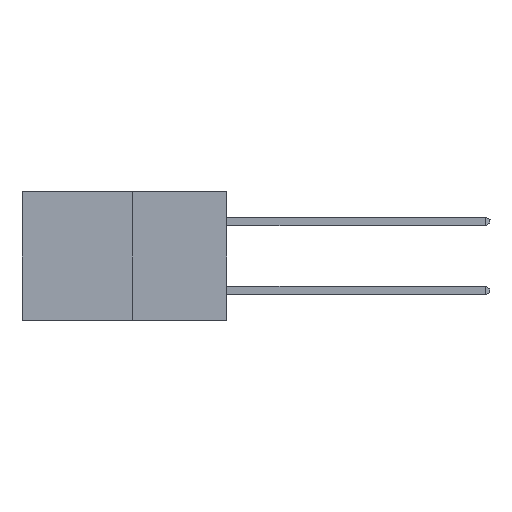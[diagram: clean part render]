
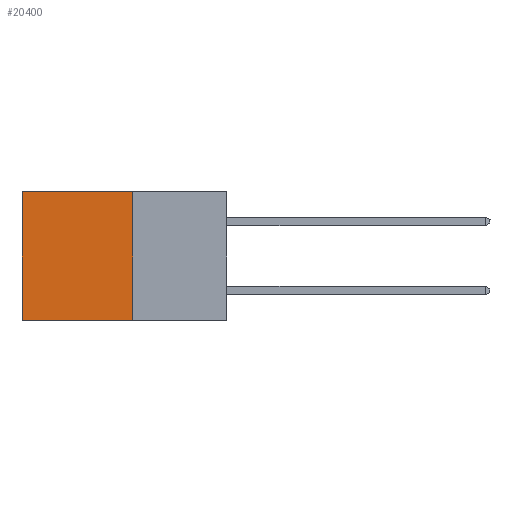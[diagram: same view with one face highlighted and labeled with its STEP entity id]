
A CAD part, left-side view. The second image highlights one B-rep face of the part: STEP entity #20400.
In plain terms, the highlighted planar face has unit normal (-1, 0, 0).
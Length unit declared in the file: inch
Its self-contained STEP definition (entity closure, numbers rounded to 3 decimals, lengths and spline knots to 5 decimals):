
#380 = CARTESIAN_POINT ( 'NONE',  ( 0.277, 0.27, -0.37 ) ) ;
#531 = VERTEX_POINT ( 'NONE', #34738 ) ;
#3915 = EDGE_CURVE ( 'NONE', #531, #27552, #3967, .T. ) ;
#3924 = ORIENTED_EDGE ( 'NONE', *, *, #5688, .T. ) ;
#3967 = LINE ( 'NONE', #10263, #10322 ) ;
#5487 = ORIENTED_EDGE ( 'NONE', *, *, #3915, .F. ) ;
#5511 = CARTESIAN_POINT ( 'NONE',  ( 0.277, 0.27, -0.37 ) ) ;
#5688 = EDGE_CURVE ( 'NONE', #26349, #24792, #20403, .T. ) ;
#5805 = EDGE_CURVE ( 'NONE', #531, #26349, #30429, .T. ) ;
#7483 = VECTOR ( 'NONE', #22074, 39.37008 ) ;
#9170 = LINE ( 'NONE', #380, #7483 ) ;
#9884 = CARTESIAN_POINT ( 'NONE',  ( 0.277, 0.27, 0. ) ) ;
#9928 = DIRECTION ( 'NONE',  ( 0., 1., 0. ) ) ;
#10263 = CARTESIAN_POINT ( 'NONE',  ( 0.277, 0.27, -0.37 ) ) ;
#10322 = VECTOR ( 'NONE', #28359, 39.37008 ) ;
#10988 = ORIENTED_EDGE ( 'NONE', *, *, #33969, .F. ) ;
#15325 = PLANE ( 'NONE',  #32573 ) ;
#16840 = DIRECTION ( 'NONE',  ( 0., 0., -1. ) ) ;
#17009 = VECTOR ( 'NONE', #9928, 39.37008 ) ;
#17057 = CARTESIAN_POINT ( 'NONE',  ( 0.277, 0.59, -0.37 ) ) ;
#18037 = DIRECTION ( 'NONE',  ( 0., 0., -1. ) ) ;
#19739 = CARTESIAN_POINT ( 'NONE',  ( 0.277, 0.59, 0. ) ) ;
#20400 = ADVANCED_FACE ( 'NONE', ( #21377 ), #15325, .F. ) ;
#20403 = LINE ( 'NONE', #17057, #33793 ) ;
#21377 = FACE_OUTER_BOUND ( 'NONE', #26515, .T. ) ;
#22074 = DIRECTION ( 'NONE',  ( 0., 1., 0. ) ) ;
#24358 = ORIENTED_EDGE ( 'NONE', *, *, #5805, .T. ) ;
#24792 = VERTEX_POINT ( 'NONE', #32463 ) ;
#25948 = CARTESIAN_POINT ( 'NONE',  ( 0.277, 0.27, -0.37 ) ) ;
#26349 = VERTEX_POINT ( 'NONE', #19739 ) ;
#26515 = EDGE_LOOP ( 'NONE', ( #3924, #10988, #5487, #24358 ) ) ;
#27552 = VERTEX_POINT ( 'NONE', #5511 ) ;
#28359 = DIRECTION ( 'NONE',  ( 0., 0., -1. ) ) ;
#30429 = LINE ( 'NONE', #9884, #17009 ) ;
#32463 = CARTESIAN_POINT ( 'NONE',  ( 0.277, 0.59, -0.37 ) ) ;
#32573 = AXIS2_PLACEMENT_3D ( 'NONE', #25948, #34083, #18037 ) ;
#33793 = VECTOR ( 'NONE', #16840, 39.37008 ) ;
#33969 = EDGE_CURVE ( 'NONE', #27552, #24792, #9170, .T. ) ;
#34083 = DIRECTION ( 'NONE',  ( 1., 0., 0. ) ) ;
#34738 = CARTESIAN_POINT ( 'NONE',  ( 0.277, 0.27, 0. ) ) ;
